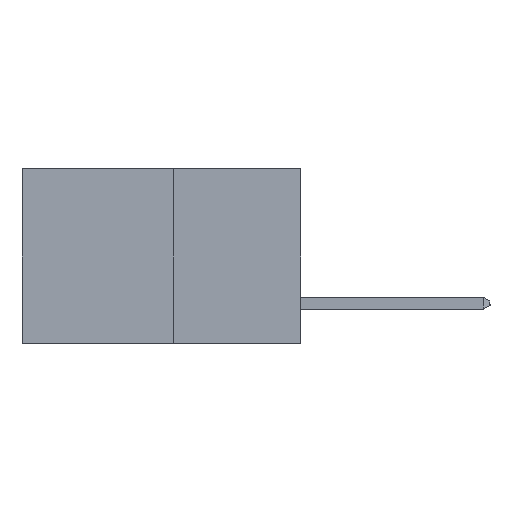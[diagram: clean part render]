
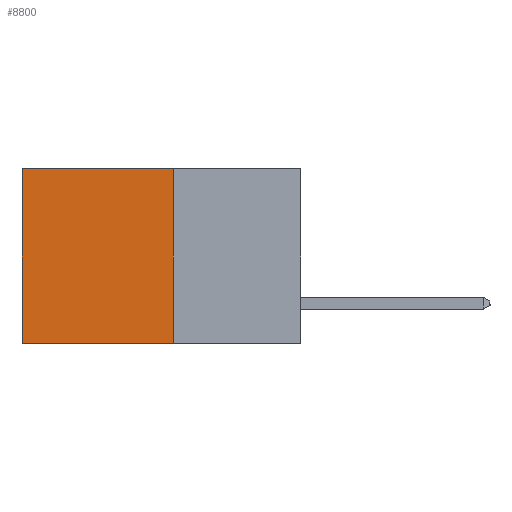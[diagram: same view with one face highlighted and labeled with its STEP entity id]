
A CAD part, left-side view. The second image highlights one B-rep face of the part: STEP entity #8800.
In plain terms, the highlighted planar face has unit normal (-1, 0, 0).
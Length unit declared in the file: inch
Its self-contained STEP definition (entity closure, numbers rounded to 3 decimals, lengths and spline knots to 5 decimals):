
#39 = CARTESIAN_POINT ( 'NONE',  ( 0.277, 0.27, -0.37 ) ) ;
#276 = CARTESIAN_POINT ( 'NONE',  ( 0.277, 0.27, -0.37 ) ) ;
#750 = CARTESIAN_POINT ( 'NONE',  ( 0.277, 0.27, 0. ) ) ;
#1296 = EDGE_CURVE ( 'NONE', #10162, #9029, #5736, .T. ) ;
#2033 = DIRECTION ( 'NONE',  ( 0., 0., -1. ) ) ;
#2462 = CARTESIAN_POINT ( 'NONE',  ( 0.277, 0.27, -0.37 ) ) ;
#2480 = AXIS2_PLACEMENT_3D ( 'NONE', #6240, #6286, #13431 ) ;
#2892 = ORIENTED_EDGE ( 'NONE', *, *, #9342, .T. ) ;
#3851 = DIRECTION ( 'NONE',  ( 0., 0., -1. ) ) ;
#4103 = VECTOR ( 'NONE', #12247, 39.37008 ) ;
#4165 = CARTESIAN_POINT ( 'NONE',  ( 0.277, 0.59, 0. ) ) ;
#5119 = FACE_OUTER_BOUND ( 'NONE', #8312, .T. ) ;
#5187 = EDGE_CURVE ( 'NONE', #9029, #7919, #8559, .T. ) ;
#5718 = ORIENTED_EDGE ( 'NONE', *, *, #10783, .T. ) ;
#5736 = LINE ( 'NONE', #2462, #10931 ) ;
#5766 = ORIENTED_EDGE ( 'NONE', *, *, #1296, .F. ) ;
#6240 = CARTESIAN_POINT ( 'NONE',  ( 0.277, 0.27, -0.37 ) ) ;
#6286 = DIRECTION ( 'NONE',  ( 1., 0., 0. ) ) ;
#6812 = CARTESIAN_POINT ( 'NONE',  ( 0.277, 0.27, 0. ) ) ;
#6867 = LINE ( 'NONE', #750, #4103 ) ;
#7295 = VECTOR ( 'NONE', #3851, 39.37008 ) ;
#7620 = LINE ( 'NONE', #10074, #7295 ) ;
#7919 = VERTEX_POINT ( 'NONE', #12151 ) ;
#8142 = VERTEX_POINT ( 'NONE', #4165 ) ;
#8312 = EDGE_LOOP ( 'NONE', ( #5718, #12648, #5766, #2892 ) ) ;
#8321 = PLANE ( 'NONE',  #2480 ) ;
#8559 = LINE ( 'NONE', #39, #11607 ) ;
#8800 = ADVANCED_FACE ( 'NONE', ( #5119 ), #8321, .F. ) ;
#8872 = DIRECTION ( 'NONE',  ( 0., 1., 0. ) ) ;
#9029 = VERTEX_POINT ( 'NONE', #276 ) ;
#9342 = EDGE_CURVE ( 'NONE', #10162, #8142, #6867, .T. ) ;
#10074 = CARTESIAN_POINT ( 'NONE',  ( 0.277, 0.59, -0.37 ) ) ;
#10162 = VERTEX_POINT ( 'NONE', #6812 ) ;
#10783 = EDGE_CURVE ( 'NONE', #8142, #7919, #7620, .T. ) ;
#10931 = VECTOR ( 'NONE', #2033, 39.37008 ) ;
#11607 = VECTOR ( 'NONE', #8872, 39.37008 ) ;
#12151 = CARTESIAN_POINT ( 'NONE',  ( 0.277, 0.59, -0.37 ) ) ;
#12247 = DIRECTION ( 'NONE',  ( 0., 1., 0. ) ) ;
#12648 = ORIENTED_EDGE ( 'NONE', *, *, #5187, .F. ) ;
#13431 = DIRECTION ( 'NONE',  ( 0., 0., -1. ) ) ;
